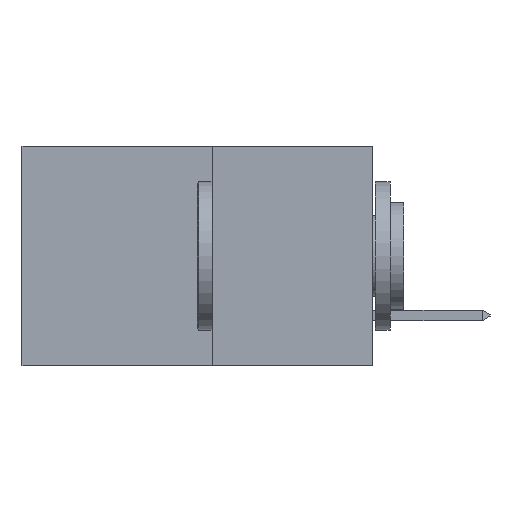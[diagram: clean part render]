
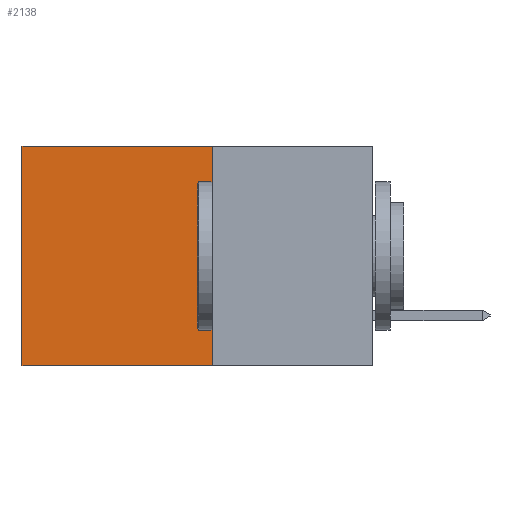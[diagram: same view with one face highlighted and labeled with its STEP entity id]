
A CAD part, left-side view. The second image highlights one B-rep face of the part: STEP entity #2138.
In plain terms, the highlighted planar face has unit normal (-1, 0, 0).
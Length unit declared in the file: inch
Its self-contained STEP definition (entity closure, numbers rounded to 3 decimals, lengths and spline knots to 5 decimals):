
#556 = DIRECTION ( 'NONE',  ( 0., 0., -1. ) ) ;
#901 = CARTESIAN_POINT ( 'NONE',  ( 0.277, 0.59, -0.37 ) ) ;
#1061 = CARTESIAN_POINT ( 'NONE',  ( 0.277, 0.27, 0. ) ) ;
#1089 = DIRECTION ( 'NONE',  ( 0., 1., 0. ) ) ;
#1552 = AXIS2_PLACEMENT_3D ( 'NONE', #7127, #5404, #6395 ) ;
#1875 = VECTOR ( 'NONE', #556, 39.37008 ) ;
#1979 = EDGE_CURVE ( 'NONE', #3231, #3013, #3416, .T. ) ;
#2002 = LINE ( 'NONE', #1061, #7408 ) ;
#2089 = CARTESIAN_POINT ( 'NONE',  ( 0.277, 0.59, -0.37 ) ) ;
#2138 = ADVANCED_FACE ( 'NONE', ( #2248 ), #5058, .F. ) ;
#2248 = FACE_OUTER_BOUND ( 'NONE', #8853, .T. ) ;
#2532 = EDGE_CURVE ( 'NONE', #5898, #3231, #2002, .T. ) ;
#2743 = EDGE_CURVE ( 'NONE', #5898, #7163, #3871, .T. ) ;
#3013 = VERTEX_POINT ( 'NONE', #901 ) ;
#3231 = VERTEX_POINT ( 'NONE', #8826 ) ;
#3276 = EDGE_CURVE ( 'NONE', #7163, #3013, #9114, .T. ) ;
#3416 = LINE ( 'NONE', #2089, #9007 ) ;
#3871 = LINE ( 'NONE', #7789, #1875 ) ;
#4583 = ORIENTED_EDGE ( 'NONE', *, *, #2532, .T. ) ;
#5058 = PLANE ( 'NONE',  #1552 ) ;
#5114 = CARTESIAN_POINT ( 'NONE',  ( 0.277, 0.27, 0. ) ) ;
#5404 = DIRECTION ( 'NONE',  ( 1., 0., 0. ) ) ;
#5718 = CARTESIAN_POINT ( 'NONE',  ( 0.277, 0.27, -0.37 ) ) ;
#5819 = ORIENTED_EDGE ( 'NONE', *, *, #2743, .F. ) ;
#5898 = VERTEX_POINT ( 'NONE', #5114 ) ;
#6170 = ORIENTED_EDGE ( 'NONE', *, *, #1979, .T. ) ;
#6395 = DIRECTION ( 'NONE',  ( 0., 0., -1. ) ) ;
#6860 = ORIENTED_EDGE ( 'NONE', *, *, #3276, .F. ) ;
#6963 = VECTOR ( 'NONE', #8204, 39.37008 ) ;
#7127 = CARTESIAN_POINT ( 'NONE',  ( 0.277, 0.27, -0.37 ) ) ;
#7163 = VERTEX_POINT ( 'NONE', #5718 ) ;
#7373 = DIRECTION ( 'NONE',  ( 0., 0., -1. ) ) ;
#7408 = VECTOR ( 'NONE', #1089, 39.37008 ) ;
#7789 = CARTESIAN_POINT ( 'NONE',  ( 0.277, 0.27, -0.37 ) ) ;
#8204 = DIRECTION ( 'NONE',  ( 0., 1., 0. ) ) ;
#8826 = CARTESIAN_POINT ( 'NONE',  ( 0.277, 0.59, 0. ) ) ;
#8853 = EDGE_LOOP ( 'NONE', ( #6170, #6860, #5819, #4583 ) ) ;
#8925 = CARTESIAN_POINT ( 'NONE',  ( 0.277, 0.27, -0.37 ) ) ;
#9007 = VECTOR ( 'NONE', #7373, 39.37008 ) ;
#9114 = LINE ( 'NONE', #8925, #6963 ) ;
